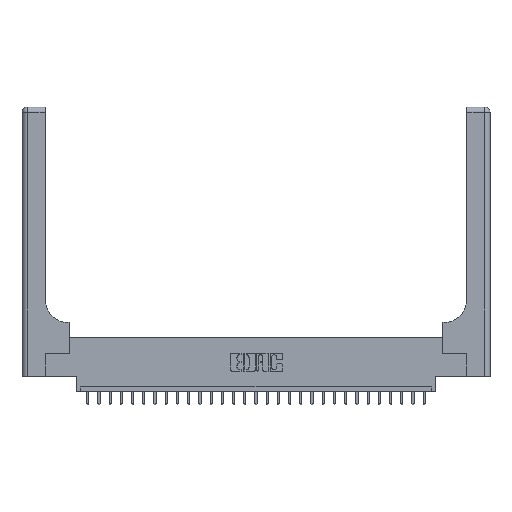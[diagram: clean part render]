
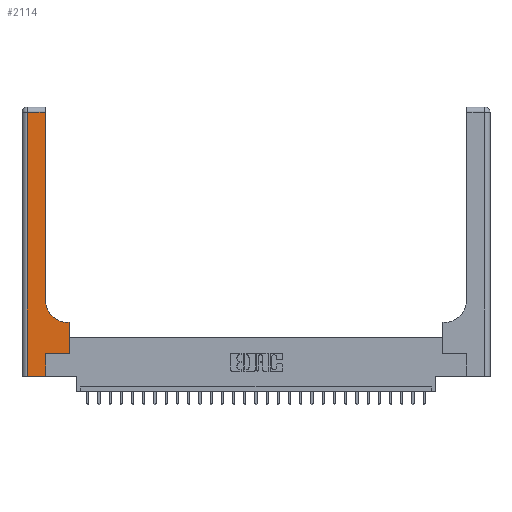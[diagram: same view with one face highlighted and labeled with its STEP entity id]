
A CAD part, top view. The second image highlights one B-rep face of the part: STEP entity #2114.
In plain terms, the highlighted planar face has unit normal (0, 0, 1).
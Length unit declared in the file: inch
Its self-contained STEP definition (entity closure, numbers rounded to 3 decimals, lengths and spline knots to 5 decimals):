
#432 = PLANE ( 'NONE',  #25712 ) ;
#533 = CARTESIAN_POINT ( 'NONE',  ( 0.06, 3., 0.37 ) ) ;
#661 = EDGE_CURVE ( 'NONE', #2762, #7952, #13599, .T. ) ;
#729 = VECTOR ( 'NONE', #11448, 39.37008 ) ;
#1233 = CARTESIAN_POINT ( 'NONE',  ( 0.26, 0.85, 0.37 ) ) ;
#1721 = CARTESIAN_POINT ( 'NONE',  ( 0.265, 0.25, 0.37 ) ) ;
#2018 = ORIENTED_EDGE ( 'NONE', *, *, #22629, .T. ) ;
#2114 = ADVANCED_FACE ( 'NONE', ( #4329 ), #432, .F. ) ;
#2299 = DIRECTION ( 'NONE',  ( -1., 0., 0. ) ) ;
#2762 = VERTEX_POINT ( 'NONE', #1721 ) ;
#2961 = AXIS2_PLACEMENT_3D ( 'NONE', #9346, #25535, #21378 ) ;
#3298 = LINE ( 'NONE', #5169, #7043 ) ;
#3444 = VERTEX_POINT ( 'NONE', #1233 ) ;
#3956 = CARTESIAN_POINT ( 'NONE',  ( 0.265, 0., 0.37 ) ) ;
#4115 = EDGE_CURVE ( 'NONE', #3444, #13864, #19109, .T. ) ;
#4329 = FACE_OUTER_BOUND ( 'NONE', #10119, .T. ) ;
#4437 = DIRECTION ( 'NONE',  ( 0., -1., 0. ) ) ;
#4463 = DIRECTION ( 'NONE',  ( -1., 0., 0. ) ) ;
#4581 = DIRECTION ( 'NONE',  ( 0., 1., 0. ) ) ;
#4767 = ORIENTED_EDGE ( 'NONE', *, *, #7467, .T. ) ;
#4911 = ORIENTED_EDGE ( 'NONE', *, *, #4115, .T. ) ;
#5169 = CARTESIAN_POINT ( 'NONE',  ( 0.265, 0., 0.37 ) ) ;
#5687 = VERTEX_POINT ( 'NONE', #12407 ) ;
#6471 = CARTESIAN_POINT ( 'NONE',  ( 0., 3., 0.37 ) ) ;
#6812 = DIRECTION ( 'NONE',  ( 0., 1., 0. ) ) ;
#6873 = EDGE_CURVE ( 'NONE', #17494, #2762, #3298, .T. ) ;
#7043 = VECTOR ( 'NONE', #25781, 39.37008 ) ;
#7070 = CARTESIAN_POINT ( 'NONE',  ( 0.06, 0., 0.37 ) ) ;
#7467 = EDGE_CURVE ( 'NONE', #7952, #20592, #18764, .T. ) ;
#7952 = VERTEX_POINT ( 'NONE', #20969 ) ;
#8000 = VECTOR ( 'NONE', #4437, 39.37008 ) ;
#8055 = EDGE_CURVE ( 'NONE', #18818, #3444, #24349, .T. ) ;
#8394 = ORIENTED_EDGE ( 'NONE', *, *, #13670, .T. ) ;
#8957 = CARTESIAN_POINT ( 'NONE',  ( 0.26, 3., 0.37 ) ) ;
#9346 = CARTESIAN_POINT ( 'NONE',  ( 0.51, 0.85, 0.37 ) ) ;
#9616 = ORIENTED_EDGE ( 'NONE', *, *, #6873, .T. ) ;
#10119 = EDGE_LOOP ( 'NONE', ( #4911, #13007, #21003, #8394, #9616, #22799, #4767, #2018, #20240 ) ) ;
#10336 = CARTESIAN_POINT ( 'NONE',  ( 0.528, 0.25, 0.37 ) ) ;
#11267 = EDGE_CURVE ( 'NONE', #13864, #5687, #20649, .T. ) ;
#11448 = DIRECTION ( 'NONE',  ( 1., 0., 0. ) ) ;
#12407 = CARTESIAN_POINT ( 'NONE',  ( 0.06, 2.94, 0.37 ) ) ;
#12855 = LINE ( 'NONE', #25040, #20341 ) ;
#13007 = ORIENTED_EDGE ( 'NONE', *, *, #11267, .T. ) ;
#13599 = LINE ( 'NONE', #17486, #15124 ) ;
#13670 = EDGE_CURVE ( 'NONE', #23204, #17494, #17600, .T. ) ;
#13864 = VERTEX_POINT ( 'NONE', #20118 ) ;
#15124 = VECTOR ( 'NONE', #25646, 39.37008 ) ;
#17486 = CARTESIAN_POINT ( 'NONE',  ( 0.265, 0.25, 0.37 ) ) ;
#17494 = VERTEX_POINT ( 'NONE', #3956 ) ;
#17600 = LINE ( 'NONE', #17867, #729 ) ;
#17867 = CARTESIAN_POINT ( 'NONE',  ( 0., 0., 0.37 ) ) ;
#18097 = VECTOR ( 'NONE', #6812, 39.37008 ) ;
#18645 = CARTESIAN_POINT ( 'NONE',  ( 0., 2.94, 0.37 ) ) ;
#18764 = LINE ( 'NONE', #10336, #21193 ) ;
#18818 = VERTEX_POINT ( 'NONE', #23099 ) ;
#19109 = LINE ( 'NONE', #8957, #18097 ) ;
#19449 = CARTESIAN_POINT ( 'NONE',  ( 0.528, 0.6, 0.37 ) ) ;
#20118 = CARTESIAN_POINT ( 'NONE',  ( 0.26, 2.94, 0.37 ) ) ;
#20240 = ORIENTED_EDGE ( 'NONE', *, *, #8055, .T. ) ;
#20341 = VECTOR ( 'NONE', #23295, 39.37008 ) ;
#20592 = VERTEX_POINT ( 'NONE', #19449 ) ;
#20649 = LINE ( 'NONE', #18645, #24055 ) ;
#20969 = CARTESIAN_POINT ( 'NONE',  ( 0.528, 0.25, 0.37 ) ) ;
#21003 = ORIENTED_EDGE ( 'NONE', *, *, #25119, .T. ) ;
#21193 = VECTOR ( 'NONE', #4581, 39.37008 ) ;
#21378 = DIRECTION ( 'NONE',  ( 1., 0., 0. ) ) ;
#22629 = EDGE_CURVE ( 'NONE', #20592, #18818, #12855, .T. ) ;
#22799 = ORIENTED_EDGE ( 'NONE', *, *, #661, .T. ) ;
#22804 = DIRECTION ( 'NONE',  ( 0., 0., -1. ) ) ;
#22914 = LINE ( 'NONE', #533, #8000 ) ;
#23099 = CARTESIAN_POINT ( 'NONE',  ( 0.51, 0.6, 0.37 ) ) ;
#23204 = VERTEX_POINT ( 'NONE', #7070 ) ;
#23295 = DIRECTION ( 'NONE',  ( -1., 0., 0. ) ) ;
#24055 = VECTOR ( 'NONE', #2299, 39.37008 ) ;
#24349 = CIRCLE ( 'NONE', #2961, 0.25 ) ;
#25040 = CARTESIAN_POINT ( 'NONE',  ( 0.26, 0.6, 0.37 ) ) ;
#25119 = EDGE_CURVE ( 'NONE', #5687, #23204, #22914, .T. ) ;
#25535 = DIRECTION ( 'NONE',  ( 0., 0., -1. ) ) ;
#25646 = DIRECTION ( 'NONE',  ( 1., 0., 0. ) ) ;
#25712 = AXIS2_PLACEMENT_3D ( 'NONE', #6471, #22804, #4463 ) ;
#25781 = DIRECTION ( 'NONE',  ( 0., 1., 0. ) ) ;
